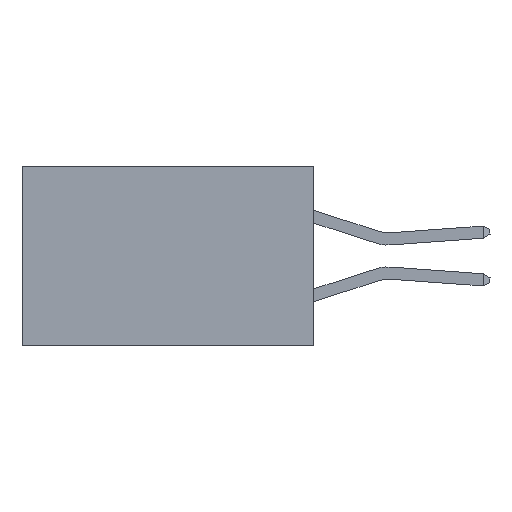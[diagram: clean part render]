
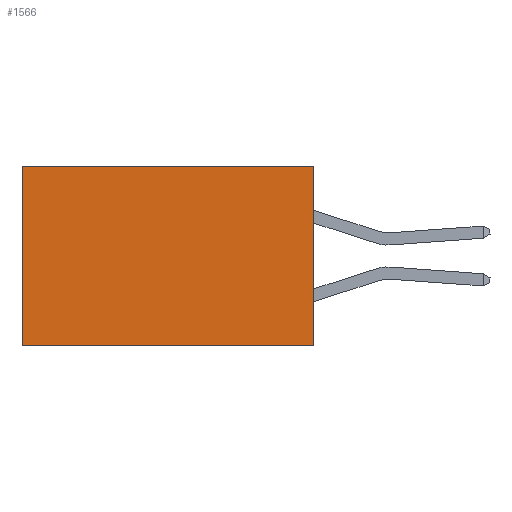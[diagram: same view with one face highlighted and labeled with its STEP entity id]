
A CAD part, left-side view. The second image highlights one B-rep face of the part: STEP entity #1566.
In plain terms, the highlighted planar face has unit normal (-1, 0, 0).
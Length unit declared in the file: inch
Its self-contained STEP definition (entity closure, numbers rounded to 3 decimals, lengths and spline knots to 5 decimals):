
#1188 = EDGE_CURVE ( 'NONE', #19071, #17365, #1359, .T. ) ;
#1339 = CARTESIAN_POINT ( 'NONE',  ( 0.2875, 0., 0. ) ) ;
#1359 = LINE ( 'NONE', #25877, #20555 ) ;
#1566 = ADVANCED_FACE ( 'NONE', ( #3032 ), #18637, .F. ) ;
#1798 = DIRECTION ( 'NONE',  ( 0., 1., 0. ) ) ;
#1799 = DIRECTION ( 'NONE',  ( 1., 0., 0. ) ) ;
#2239 = CARTESIAN_POINT ( 'NONE',  ( 0.2875, 0., -0.37 ) ) ;
#3032 = FACE_OUTER_BOUND ( 'NONE', #23630, .T. ) ;
#3260 = ORIENTED_EDGE ( 'NONE', *, *, #7280, .F. ) ;
#7280 = EDGE_CURVE ( 'NONE', #19071, #32865, #29490, .T. ) ;
#7408 = ORIENTED_EDGE ( 'NONE', *, *, #12992, .F. ) ;
#7728 = ORIENTED_EDGE ( 'NONE', *, *, #1188, .T. ) ;
#9223 = DIRECTION ( 'NONE',  ( 0., 1., 0. ) ) ;
#9897 = CARTESIAN_POINT ( 'NONE',  ( 0.2875, 0., 0. ) ) ;
#12992 = EDGE_CURVE ( 'NONE', #32865, #26288, #16130, .T. ) ;
#15391 = CARTESIAN_POINT ( 'NONE',  ( 0.2875, 0.6, -0.37 ) ) ;
#15920 = VECTOR ( 'NONE', #32300, 39.37008 ) ;
#16130 = LINE ( 'NONE', #2239, #18312 ) ;
#16790 = DIRECTION ( 'NONE',  ( 0., 0., -1. ) ) ;
#16848 = EDGE_CURVE ( 'NONE', #17365, #26288, #27645, .T. ) ;
#17365 = VERTEX_POINT ( 'NONE', #35945 ) ;
#18312 = VECTOR ( 'NONE', #1798, 39.37008 ) ;
#18637 = PLANE ( 'NONE',  #30221 ) ;
#19071 = VERTEX_POINT ( 'NONE', #1339 ) ;
#19238 = CARTESIAN_POINT ( 'NONE',  ( 0.2875, 0., 0. ) ) ;
#20555 = VECTOR ( 'NONE', #9223, 39.37008 ) ;
#23630 = EDGE_LOOP ( 'NONE', ( #32659, #7408, #3260, #7728 ) ) ;
#24096 = DIRECTION ( 'NONE',  ( 0., 0., -1. ) ) ;
#25556 = CARTESIAN_POINT ( 'NONE',  ( 0.2875, 0., -0.37 ) ) ;
#25877 = CARTESIAN_POINT ( 'NONE',  ( 0.2875, 0., 0. ) ) ;
#26288 = VERTEX_POINT ( 'NONE', #15391 ) ;
#27645 = LINE ( 'NONE', #29794, #15920 ) ;
#28144 = VECTOR ( 'NONE', #16790, 39.37008 ) ;
#29490 = LINE ( 'NONE', #19238, #28144 ) ;
#29794 = CARTESIAN_POINT ( 'NONE',  ( 0.2875, 0.6, 0. ) ) ;
#30221 = AXIS2_PLACEMENT_3D ( 'NONE', #9897, #1799, #24096 ) ;
#32300 = DIRECTION ( 'NONE',  ( 0., 0., -1. ) ) ;
#32659 = ORIENTED_EDGE ( 'NONE', *, *, #16848, .T. ) ;
#32865 = VERTEX_POINT ( 'NONE', #25556 ) ;
#35945 = CARTESIAN_POINT ( 'NONE',  ( 0.2875, 0.6, 0. ) ) ;
